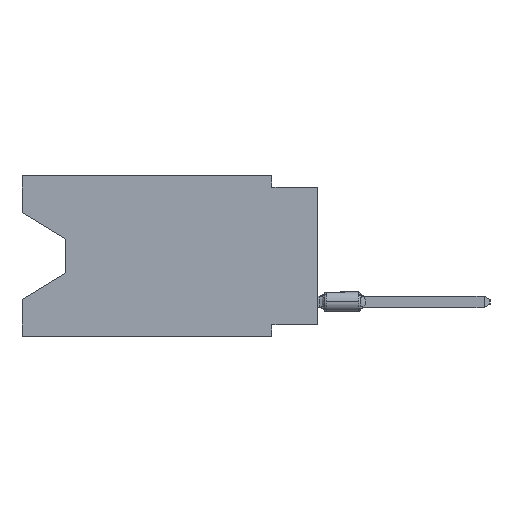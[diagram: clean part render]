
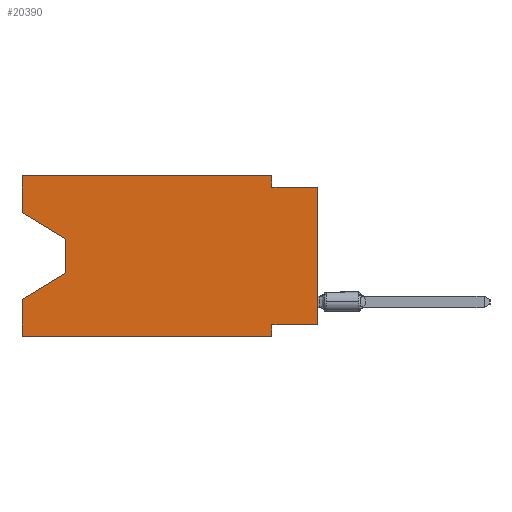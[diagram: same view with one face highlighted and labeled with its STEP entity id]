
A CAD part, left-side view. The second image highlights one B-rep face of the part: STEP entity #20390.
In plain terms, the highlighted planar face has unit normal (-1, 0, 0).
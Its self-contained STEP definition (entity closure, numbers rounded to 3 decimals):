
#278 = LINE ( 'NONE', #13409, #50754 ) ;
#1195 = CARTESIAN_POINT ( 'NONE',  ( 0., 2.54, 0. ) ) ;
#2468 = DIRECTION ( 'NONE',  ( 0., 0., -1. ) ) ;
#2578 = EDGE_CURVE ( 'NONE', #27115, #16180, #24550, .T. ) ;
#2667 = ORIENTED_EDGE ( 'NONE', *, *, #38047, .F. ) ;
#3102 = DIRECTION ( 'NONE',  ( 0., 0., -1. ) ) ;
#3125 = DIRECTION ( 'NONE',  ( 0., 0., 1. ) ) ;
#3691 = VERTEX_POINT ( 'NONE', #7446 ) ;
#3960 = ORIENTED_EDGE ( 'NONE', *, *, #23596, .F. ) ;
#4558 = CARTESIAN_POINT ( 'NONE',  ( 0., 2.54, 0. ) ) ;
#4835 = CARTESIAN_POINT ( 'NONE',  ( 0., 16.383, 0. ) ) ;
#6704 = ORIENTED_EDGE ( 'NONE', *, *, #54827, .T. ) ;
#7150 = EDGE_CURVE ( 'NONE', #41903, #8991, #40847, .T. ) ;
#7219 = ORIENTED_EDGE ( 'NONE', *, *, #33258, .F. ) ;
#7349 = VERTEX_POINT ( 'NONE', #20158 ) ;
#7446 = CARTESIAN_POINT ( 'NONE',  ( 0., 13.97, -5.385 ) ) ;
#7918 = VERTEX_POINT ( 'NONE', #47711 ) ;
#8042 = ORIENTED_EDGE ( 'NONE', *, *, #15814, .T. ) ;
#8276 = DIRECTION ( 'NONE',  ( 0., -1., 0. ) ) ;
#8595 = ORIENTED_EDGE ( 'NONE', *, *, #49818, .T. ) ;
#8991 = VERTEX_POINT ( 'NONE', #43523 ) ;
#10039 = DIRECTION ( 'NONE',  ( 1., 0., 0. ) ) ;
#10668 = DIRECTION ( 'NONE',  ( 0., 0., -1. ) ) ;
#11046 = VERTEX_POINT ( 'NONE', #35130 ) ;
#11987 = DIRECTION ( 'NONE',  ( 0., 0., 1. ) ) ;
#12753 = VECTOR ( 'NONE', #8276, 1000. ) ;
#13409 = CARTESIAN_POINT ( 'NONE',  ( 0., 16.383, -2.038 ) ) ;
#13680 = ORIENTED_EDGE ( 'NONE', *, *, #43734, .T. ) ;
#14138 = ORIENTED_EDGE ( 'NONE', *, *, #44655, .F. ) ;
#14354 = DIRECTION ( 'NONE',  ( 0., 1., 0. ) ) ;
#14656 = LINE ( 'NONE', #30869, #30013 ) ;
#15814 = EDGE_CURVE ( 'NONE', #27115, #8991, #14656, .T. ) ;
#16180 = VERTEX_POINT ( 'NONE', #27280 ) ;
#17373 = ORIENTED_EDGE ( 'NONE', *, *, #2578, .F. ) ;
#18785 = CARTESIAN_POINT ( 'NONE',  ( 0., 2.54, -8.89 ) ) ;
#19374 = VECTOR ( 'NONE', #45289, 1000. ) ;
#19715 = VERTEX_POINT ( 'NONE', #26396 ) ;
#20158 = CARTESIAN_POINT ( 'NONE',  ( 0., 2.54, -0.635 ) ) ;
#20390 = ADVANCED_FACE ( 'NONE', ( #23990 ), #48304, .F. ) ;
#20700 = LINE ( 'NONE', #41947, #19374 ) ;
#22352 = AXIS2_PLACEMENT_3D ( 'NONE', #27070, #10039, #2468 ) ;
#23492 = EDGE_LOOP ( 'NONE', ( #48131, #8595, #13680, #17373, #8042, #42099, #7219, #6704, #3960, #2667, #14138, #50838 ) ) ;
#23596 = EDGE_CURVE ( 'NONE', #7349, #19715, #50446, .T. ) ;
#23990 = FACE_OUTER_BOUND ( 'NONE', #23492, .T. ) ;
#24550 = LINE ( 'NONE', #50262, #41605 ) ;
#26396 = CARTESIAN_POINT ( 'NONE',  ( 0., 0., -0.635 ) ) ;
#27070 = CARTESIAN_POINT ( 'NONE',  ( 0., 16.383, 0. ) ) ;
#27115 = VERTEX_POINT ( 'NONE', #40143 ) ;
#27280 = CARTESIAN_POINT ( 'NONE',  ( 0., 16.383, -6.852 ) ) ;
#28540 = CARTESIAN_POINT ( 'NONE',  ( 0., 13.97, -3.505 ) ) ;
#28658 = CARTESIAN_POINT ( 'NONE',  ( 0., 0., -0.635 ) ) ;
#28807 = LINE ( 'NONE', #50605, #29342 ) ;
#29342 = VECTOR ( 'NONE', #38043, 1000. ) ;
#29407 = CARTESIAN_POINT ( 'NONE',  ( 0., 0., 0. ) ) ;
#29985 = LINE ( 'NONE', #4835, #33786 ) ;
#30013 = VECTOR ( 'NONE', #47910, 1000. ) ;
#30869 = CARTESIAN_POINT ( 'NONE',  ( 0., 16.383, -8.89 ) ) ;
#31134 = CARTESIAN_POINT ( 'NONE',  ( 0., 2.54, -8.255 ) ) ;
#32889 = CARTESIAN_POINT ( 'NONE',  ( 0., 0., -8.255 ) ) ;
#32899 = VECTOR ( 'NONE', #39758, 1000. ) ;
#33258 = EDGE_CURVE ( 'NONE', #40176, #41903, #35023, .T. ) ;
#33786 = VECTOR ( 'NONE', #43928, 1000. ) ;
#35023 = LINE ( 'NONE', #52610, #47719 ) ;
#35130 = CARTESIAN_POINT ( 'NONE',  ( 0., 16.383, -2.038 ) ) ;
#35920 = CARTESIAN_POINT ( 'NONE',  ( 0., 13.97, -3.505 ) ) ;
#38043 = DIRECTION ( 'NONE',  ( 0., 0., 1. ) ) ;
#38047 = EDGE_CURVE ( 'NONE', #43507, #7349, #48134, .T. ) ;
#39758 = DIRECTION ( 'NONE',  ( 0., 0., -1. ) ) ;
#40143 = CARTESIAN_POINT ( 'NONE',  ( 0., 16.383, -8.89 ) ) ;
#40176 = VERTEX_POINT ( 'NONE', #32889 ) ;
#40489 = VERTEX_POINT ( 'NONE', #35920 ) ;
#40847 = LINE ( 'NONE', #18785, #51642 ) ;
#41605 = VECTOR ( 'NONE', #11987, 1000. ) ;
#41903 = VERTEX_POINT ( 'NONE', #31134 ) ;
#41947 = CARTESIAN_POINT ( 'NONE',  ( 0., 13.97, -5.385 ) ) ;
#42099 = ORIENTED_EDGE ( 'NONE', *, *, #7150, .F. ) ;
#43507 = VERTEX_POINT ( 'NONE', #4558 ) ;
#43523 = CARTESIAN_POINT ( 'NONE',  ( 0., 2.54, -8.89 ) ) ;
#43734 = EDGE_CURVE ( 'NONE', #3691, #16180, #20700, .T. ) ;
#43928 = DIRECTION ( 'NONE',  ( 0., -1., 0. ) ) ;
#44655 = EDGE_CURVE ( 'NONE', #7918, #43507, #29985, .T. ) ;
#44978 = EDGE_CURVE ( 'NONE', #11046, #7918, #28807, .T. ) ;
#45289 = DIRECTION ( 'NONE',  ( 0., 0.855, -0.519 ) ) ;
#46242 = EDGE_CURVE ( 'NONE', #11046, #40489, #278, .T. ) ;
#47711 = CARTESIAN_POINT ( 'NONE',  ( 0., 16.383, 0. ) ) ;
#47719 = VECTOR ( 'NONE', #14354, 1000. ) ;
#47910 = DIRECTION ( 'NONE',  ( 0., -1., 0. ) ) ;
#48131 = ORIENTED_EDGE ( 'NONE', *, *, #46242, .T. ) ;
#48134 = LINE ( 'NONE', #1195, #32899 ) ;
#48304 = PLANE ( 'NONE',  #22352 ) ;
#49081 = VECTOR ( 'NONE', #3102, 1000. ) ;
#49212 = LINE ( 'NONE', #28540, #49081 ) ;
#49818 = EDGE_CURVE ( 'NONE', #40489, #3691, #49212, .T. ) ;
#50081 = LINE ( 'NONE', #29407, #53067 ) ;
#50262 = CARTESIAN_POINT ( 'NONE',  ( 0., 16.383, 0. ) ) ;
#50446 = LINE ( 'NONE', #28658, #12753 ) ;
#50605 = CARTESIAN_POINT ( 'NONE',  ( 0., 16.383, 0. ) ) ;
#50754 = VECTOR ( 'NONE', #50859, 1000. ) ;
#50838 = ORIENTED_EDGE ( 'NONE', *, *, #44978, .F. ) ;
#50859 = DIRECTION ( 'NONE',  ( 0., -0.855, -0.519 ) ) ;
#51642 = VECTOR ( 'NONE', #10668, 1000. ) ;
#52610 = CARTESIAN_POINT ( 'NONE',  ( 0., 0., -8.255 ) ) ;
#53067 = VECTOR ( 'NONE', #3125, 1000. ) ;
#54827 = EDGE_CURVE ( 'NONE', #40176, #19715, #50081, .T. ) ;
